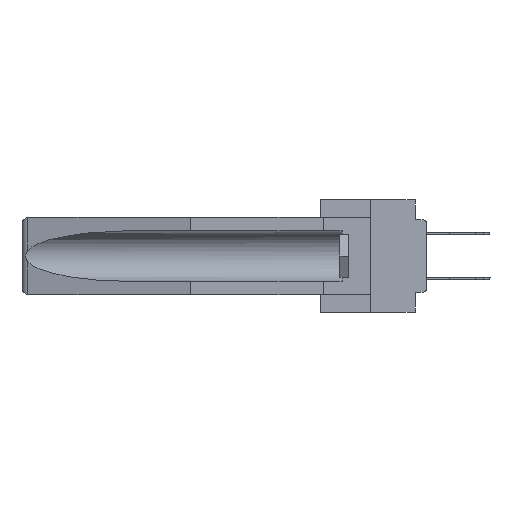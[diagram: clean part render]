
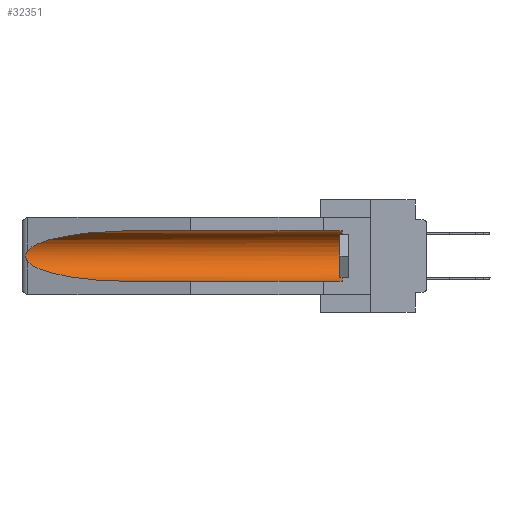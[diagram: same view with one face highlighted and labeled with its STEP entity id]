
A CAD part, left-side view. The second image highlights one B-rep face of the part: STEP entity #32351.
In plain terms, the highlighted cylindrical face has radius 2.857 mm (diameter 5.715 mm), a partial arc.
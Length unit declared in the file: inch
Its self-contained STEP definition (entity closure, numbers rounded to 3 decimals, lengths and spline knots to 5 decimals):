
#513 = CARTESIAN_POINT ( 'NONE',  ( 0.155, 0.126, -0.1715 ) ) ;
#1065 = CARTESIAN_POINT ( 'NONE',  ( 0.2673, 1.53269, -0.17917 ) ) ;
#1235 = CARTESIAN_POINT ( 'NONE',  ( 0.155, -0.30754, -0.059 ) ) ;
#1498 = EDGE_CURVE ( 'NONE', #6393, #29595, #30746, .T. ) ;
#2748 = LINE ( 'NONE', #3167, #5835 ) ;
#3167 = CARTESIAN_POINT ( 'NONE',  ( 0.155, -0.30754, -0.284 ) ) ;
#3544 = ORIENTED_EDGE ( 'NONE', *, *, #8611, .T. ) ;
#3876 = VECTOR ( 'NONE', #35789, 39.37008 ) ;
#3878 = CARTESIAN_POINT ( 'NONE',  ( 0.2673, 1.5327, -0.16383 ) ) ;
#4469 = VERTEX_POINT ( 'NONE', #36016 ) ;
#5835 = VECTOR ( 'NONE', #28817, 39.37008 ) ;
#6393 = VERTEX_POINT ( 'NONE', #33277 ) ;
#6818 = CARTESIAN_POINT ( 'NONE',  ( 0.26537, 1.52718, -0.19328 ) ) ;
#8611 = EDGE_CURVE ( 'NONE', #13761, #6393, #23653, .T. ) ;
#9193 = CARTESIAN_POINT ( 'NONE',  ( 0.155, 1.07973, -0.284 ) ) ;
#9260 = CARTESIAN_POINT ( 'NONE',  ( 0.26537, 1.52718, -0.14972 ) ) ;
#9839 =( BOUNDED_CURVE ( )  B_SPLINE_CURVE ( 3, ( #25591, #17286, #11477, #34663 ),
 .UNSPECIFIED., .F., .F. ) 
 B_SPLINE_CURVE_WITH_KNOTS ( ( 4, 4 ),
 ( 4.71239, 6.08839 ),
 .UNSPECIFIED. ) 
 CURVE ( )  GEOMETRIC_REPRESENTATION_ITEM ( )  RATIONAL_B_SPLINE_CURVE ( ( 1., 0.848, 0.848, 1. ) ) 
 REPRESENTATION_ITEM ( '' )  );
#11477 = CARTESIAN_POINT ( 'NONE',  ( 0.25451, 1.48313, -0.09465 ) ) ;
#12287 = CARTESIAN_POINT ( 'NONE',  ( 0.26654, 1.53092, -0.15636 ) ) ;
#12345 = VERTEX_POINT ( 'NONE', #28224 ) ;
#12413 = EDGE_CURVE ( 'NONE', #12345, #13761, #9839, .T. ) ;
#12786 = CARTESIAN_POINT ( 'NONE',  ( 0.26597, 1.52961, -0.15275 ) ) ;
#13073 = VERTEX_POINT ( 'NONE', #34097 ) ;
#13160 = DIRECTION ( 'NONE',  ( 0., 1., 0. ) ) ;
#13634 = LINE ( 'NONE', #1235, #3876 ) ;
#13761 = VERTEX_POINT ( 'NONE', #9260 ) ;
#15405 = CARTESIAN_POINT ( 'NONE',  ( 0.26655, 1.53094, -0.18657 ) ) ;
#17286 = CARTESIAN_POINT ( 'NONE',  ( 0.21114, 1.30732, -0.059 ) ) ;
#17436 = DIRECTION ( 'NONE',  ( 0., 0., 1. ) ) ;
#17998 = CARTESIAN_POINT ( 'NONE',  ( 0.2675, 1.53308, -0.17534 ) ) ;
#18124 = CARTESIAN_POINT ( 'NONE',  ( 0.26537, 1.52718, -0.19328 ) ) ;
#19354 = DIRECTION ( 'NONE',  ( 0., 0., 1. ) ) ;
#19737 = ORIENTED_EDGE ( 'NONE', *, *, #31532, .T. ) ;
#20455 = CARTESIAN_POINT ( 'NONE',  ( 0.25451, 1.48313, -0.24835 ) ) ;
#20865 = CARTESIAN_POINT ( 'NONE',  ( 0.26597, 1.5296, -0.19026 ) ) ;
#22907 = CYLINDRICAL_SURFACE ( 'NONE', #30063, 0.1125 ) ;
#23284 = CARTESIAN_POINT ( 'NONE',  ( 0.21114, 1.30732, -0.284 ) ) ;
#23653 = B_SPLINE_CURVE_WITH_KNOTS ( 'NONE', 3,
 ( #35387, #12786, #12287, #3878, #32146, #17998, #1065, #15405, #20865, #18124 ),
 .UNSPECIFIED., .F., .F.,
 ( 4, 2, 2, 2, 4 ),
 ( 0., 0.00029, 0.00058, 0.00087, 0.00117 ),
 .UNSPECIFIED. ) ;
#25591 = CARTESIAN_POINT ( 'NONE',  ( 0.155, 1.07973, -0.059 ) ) ;
#25719 = EDGE_LOOP ( 'NONE', ( #33617, #3544, #28317, #32644, #28415, #19737 ) ) ;
#25749 = DIRECTION ( 'NONE',  ( 0., -1., 0. ) ) ;
#27393 = AXIS2_PLACEMENT_3D ( 'NONE', #513, #25749, #17436 ) ;
#27414 = CARTESIAN_POINT ( 'NONE',  ( 0.155, -0.30754, -0.1715 ) ) ;
#28224 = CARTESIAN_POINT ( 'NONE',  ( 0.155, 1.07973, -0.059 ) ) ;
#28317 = ORIENTED_EDGE ( 'NONE', *, *, #1498, .T. ) ;
#28415 = ORIENTED_EDGE ( 'NONE', *, *, #30586, .T. ) ;
#28817 = DIRECTION ( 'NONE',  ( 0., 1., 0. ) ) ;
#29127 = EDGE_CURVE ( 'NONE', #4469, #29595, #2748, .T. ) ;
#29574 = FACE_OUTER_BOUND ( 'NONE', #25719, .T. ) ;
#29595 = VERTEX_POINT ( 'NONE', #35752 ) ;
#30063 = AXIS2_PLACEMENT_3D ( 'NONE', #27414, #13160, #19354 ) ;
#30586 = EDGE_CURVE ( 'NONE', #4469, #13073, #33204, .T. ) ;
#30746 =( BOUNDED_CURVE ( )  B_SPLINE_CURVE ( 3, ( #6818, #20455, #23284, #9193 ),
 .UNSPECIFIED., .F., .F. ) 
 B_SPLINE_CURVE_WITH_KNOTS ( ( 4, 4 ),
 ( 0.1948, 1.5708 ),
 .UNSPECIFIED. ) 
 CURVE ( )  GEOMETRIC_REPRESENTATION_ITEM ( )  RATIONAL_B_SPLINE_CURVE ( ( 1., 0.848, 0.848, 1. ) ) 
 REPRESENTATION_ITEM ( '' )  );
#31532 = EDGE_CURVE ( 'NONE', #13073, #12345, #13634, .T. ) ;
#32146 = CARTESIAN_POINT ( 'NONE',  ( 0.2675, 1.53308, -0.16763 ) ) ;
#32351 = ADVANCED_FACE ( 'NONE', ( #29574 ), #22907, .F. ) ;
#32644 = ORIENTED_EDGE ( 'NONE', *, *, #29127, .F. ) ;
#33204 = CIRCLE ( 'NONE', #27393, 0.1125 ) ;
#33277 = CARTESIAN_POINT ( 'NONE',  ( 0.26537, 1.52718, -0.19328 ) ) ;
#33617 = ORIENTED_EDGE ( 'NONE', *, *, #12413, .T. ) ;
#34097 = CARTESIAN_POINT ( 'NONE',  ( 0.155, 0.126, -0.059 ) ) ;
#34663 = CARTESIAN_POINT ( 'NONE',  ( 0.26537, 1.52718, -0.14972 ) ) ;
#35387 = CARTESIAN_POINT ( 'NONE',  ( 0.26537, 1.52718, -0.14972 ) ) ;
#35752 = CARTESIAN_POINT ( 'NONE',  ( 0.155, 1.07973, -0.284 ) ) ;
#35789 = DIRECTION ( 'NONE',  ( 0., 1., 0. ) ) ;
#36016 = CARTESIAN_POINT ( 'NONE',  ( 0.155, 0.126, -0.284 ) ) ;
